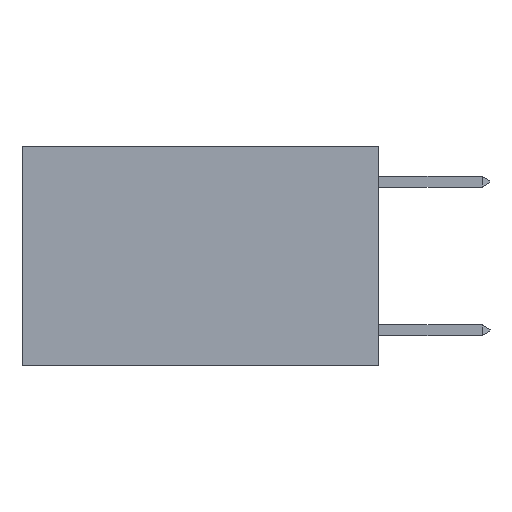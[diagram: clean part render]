
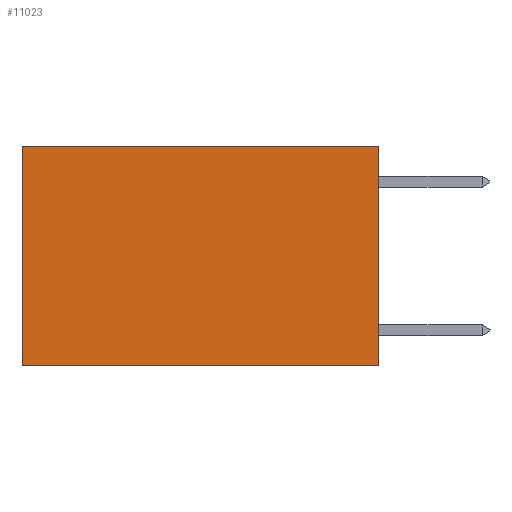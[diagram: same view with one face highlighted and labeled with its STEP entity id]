
A CAD part, left-side view. The second image highlights one B-rep face of the part: STEP entity #11023.
In plain terms, the highlighted planar face has unit normal (-1, 0, 0).
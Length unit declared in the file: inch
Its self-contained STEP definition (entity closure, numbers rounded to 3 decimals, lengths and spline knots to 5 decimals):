
#539 = EDGE_CURVE ( 'NONE', #6096, #4194, #5794, .T. ) ;
#737 = DIRECTION ( 'NONE',  ( 1., 0., 0. ) ) ;
#897 = VECTOR ( 'NONE', #9223, 39.37008 ) ;
#921 = LINE ( 'NONE', #9903, #7873 ) ;
#1622 = ORIENTED_EDGE ( 'NONE', *, *, #8632, .T. ) ;
#1735 = AXIS2_PLACEMENT_3D ( 'NONE', #11544, #737, #7113 ) ;
#1976 = CARTESIAN_POINT ( 'NONE',  ( 0.2625, 0., 0. ) ) ;
#2275 = ORIENTED_EDGE ( 'NONE', *, *, #4244, .T. ) ;
#2702 = DIRECTION ( 'NONE',  ( 0., 1., 0. ) ) ;
#3483 = VECTOR ( 'NONE', #10829, 39.37008 ) ;
#4194 = VERTEX_POINT ( 'NONE', #7266 ) ;
#4244 = EDGE_CURVE ( 'NONE', #7358, #6832, #10613, .T. ) ;
#5059 = EDGE_LOOP ( 'NONE', ( #2275, #10565, #7081, #1622 ) ) ;
#5339 = PLANE ( 'NONE',  #1735 ) ;
#5429 = CARTESIAN_POINT ( 'NONE',  ( 0.2625, 0.6, -0.37 ) ) ;
#5794 = LINE ( 'NONE', #1976, #897 ) ;
#5886 = CARTESIAN_POINT ( 'NONE',  ( 0.2625, 0., 0. ) ) ;
#5938 = VECTOR ( 'NONE', #6774, 39.37008 ) ;
#6096 = VERTEX_POINT ( 'NONE', #10048 ) ;
#6489 = LINE ( 'NONE', #5886, #5938 ) ;
#6774 = DIRECTION ( 'NONE',  ( 0., 1., 0. ) ) ;
#6832 = VERTEX_POINT ( 'NONE', #5429 ) ;
#7081 = ORIENTED_EDGE ( 'NONE', *, *, #539, .F. ) ;
#7113 = DIRECTION ( 'NONE',  ( 0., 0., -1. ) ) ;
#7266 = CARTESIAN_POINT ( 'NONE',  ( 0.2625, 0., -0.37 ) ) ;
#7358 = VERTEX_POINT ( 'NONE', #9552 ) ;
#7543 = FACE_OUTER_BOUND ( 'NONE', #5059, .T. ) ;
#7700 = EDGE_CURVE ( 'NONE', #4194, #6832, #921, .T. ) ;
#7873 = VECTOR ( 'NONE', #2702, 39.37008 ) ;
#8632 = EDGE_CURVE ( 'NONE', #6096, #7358, #6489, .T. ) ;
#9223 = DIRECTION ( 'NONE',  ( 0., 0., -1. ) ) ;
#9552 = CARTESIAN_POINT ( 'NONE',  ( 0.2625, 0.6, 0. ) ) ;
#9903 = CARTESIAN_POINT ( 'NONE',  ( 0.2625, 0., -0.37 ) ) ;
#9942 = CARTESIAN_POINT ( 'NONE',  ( 0.2625, 0.6, 0. ) ) ;
#10048 = CARTESIAN_POINT ( 'NONE',  ( 0.2625, 0., 0. ) ) ;
#10565 = ORIENTED_EDGE ( 'NONE', *, *, #7700, .F. ) ;
#10613 = LINE ( 'NONE', #9942, #3483 ) ;
#10829 = DIRECTION ( 'NONE',  ( 0., 0., -1. ) ) ;
#11023 = ADVANCED_FACE ( 'NONE', ( #7543 ), #5339, .F. ) ;
#11544 = CARTESIAN_POINT ( 'NONE',  ( 0.2625, 0., 0. ) ) ;
